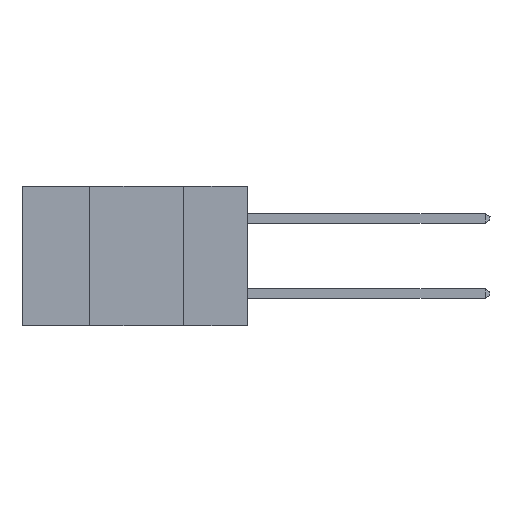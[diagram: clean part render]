
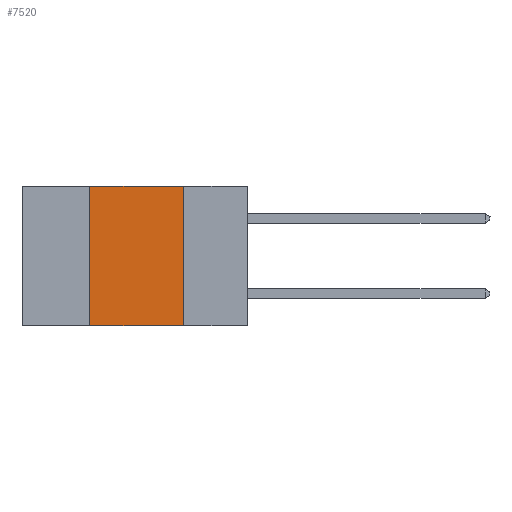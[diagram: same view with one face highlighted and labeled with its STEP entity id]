
A CAD part, left-side view. The second image highlights one B-rep face of the part: STEP entity #7520.
In plain terms, the highlighted planar face has unit normal (-1, 0, 0).
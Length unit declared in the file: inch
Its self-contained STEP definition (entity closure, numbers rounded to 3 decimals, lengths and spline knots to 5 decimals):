
#215 = AXIS2_PLACEMENT_3D ( 'NONE', #9032, #792, #859 ) ;
#342 = EDGE_CURVE ( 'NONE', #12526, #5148, #12398, .T. ) ;
#485 = VECTOR ( 'NONE', #3219, 39.37008 ) ;
#792 = DIRECTION ( 'NONE',  ( 1., 0., 0. ) ) ;
#855 = ORIENTED_EDGE ( 'NONE', *, *, #8417, .F. ) ;
#859 = DIRECTION ( 'NONE',  ( 0., 0., -1. ) ) ;
#1352 = ORIENTED_EDGE ( 'NONE', *, *, #11391, .F. ) ;
#1705 = ORIENTED_EDGE ( 'NONE', *, *, #4678, .T. ) ;
#1856 = CARTESIAN_POINT ( 'NONE',  ( 0., 0.42, 0. ) ) ;
#1990 = LINE ( 'NONE', #8107, #3735 ) ;
#2088 = EDGE_LOOP ( 'NONE', ( #855, #1352, #9719, #1705 ) ) ;
#2996 = DIRECTION ( 'NONE',  ( 0., -1., 0. ) ) ;
#3219 = DIRECTION ( 'NONE',  ( 0., 0., 1. ) ) ;
#3735 = VECTOR ( 'NONE', #2996, 39.37008 ) ;
#3822 = VERTEX_POINT ( 'NONE', #9697 ) ;
#4238 = LINE ( 'NONE', #8243, #9700 ) ;
#4244 = VECTOR ( 'NONE', #4731, 39.37008 ) ;
#4448 = VERTEX_POINT ( 'NONE', #9365 ) ;
#4678 = EDGE_CURVE ( 'NONE', #12526, #4448, #1990, .T. ) ;
#4731 = DIRECTION ( 'NONE',  ( 0., 0., -1. ) ) ;
#5148 = VERTEX_POINT ( 'NONE', #1856 ) ;
#6614 = LINE ( 'NONE', #12573, #4244 ) ;
#6741 = FACE_OUTER_BOUND ( 'NONE', #2088, .T. ) ;
#7411 = CARTESIAN_POINT ( 'NONE',  ( 0., 0.42, -0.37 ) ) ;
#7520 = ADVANCED_FACE ( 'NONE', ( #6741 ), #10045, .F. ) ;
#8107 = CARTESIAN_POINT ( 'NONE',  ( 0., 0.6, -0.37 ) ) ;
#8243 = CARTESIAN_POINT ( 'NONE',  ( 0., 0.6, 0. ) ) ;
#8417 = EDGE_CURVE ( 'NONE', #3822, #4448, #6614, .T. ) ;
#8461 = CARTESIAN_POINT ( 'NONE',  ( 0., 0.42, -0.37 ) ) ;
#9032 = CARTESIAN_POINT ( 'NONE',  ( 0., 0.6, 0. ) ) ;
#9365 = CARTESIAN_POINT ( 'NONE',  ( 0., 0.17, -0.37 ) ) ;
#9697 = CARTESIAN_POINT ( 'NONE',  ( 0., 0.17, 0. ) ) ;
#9700 = VECTOR ( 'NONE', #12232, 39.37008 ) ;
#9719 = ORIENTED_EDGE ( 'NONE', *, *, #342, .F. ) ;
#10045 = PLANE ( 'NONE',  #215 ) ;
#11391 = EDGE_CURVE ( 'NONE', #5148, #3822, #4238, .T. ) ;
#12232 = DIRECTION ( 'NONE',  ( 0., -1., 0. ) ) ;
#12398 = LINE ( 'NONE', #7411, #485 ) ;
#12526 = VERTEX_POINT ( 'NONE', #8461 ) ;
#12573 = CARTESIAN_POINT ( 'NONE',  ( 0., 0.17, -0.37 ) ) ;
